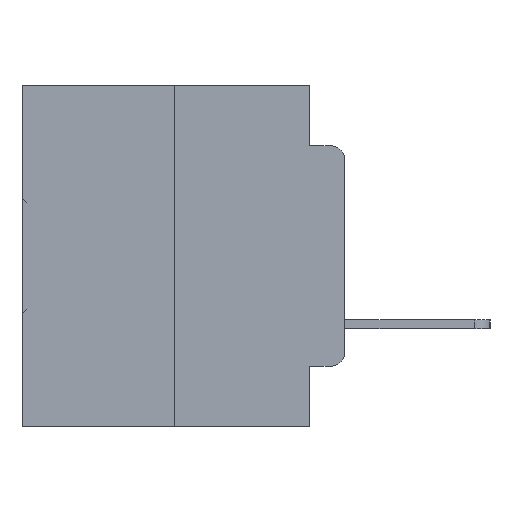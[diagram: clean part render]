
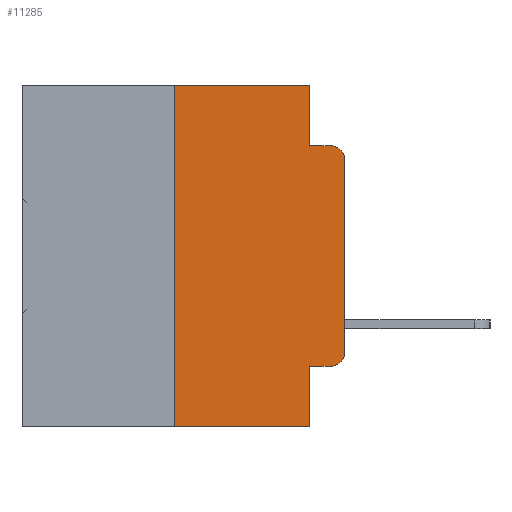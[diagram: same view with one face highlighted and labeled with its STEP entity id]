
A CAD part, left-side view. The second image highlights one B-rep face of the part: STEP entity #11285.
In plain terms, the highlighted planar face has unit normal (-1, 0, 0).
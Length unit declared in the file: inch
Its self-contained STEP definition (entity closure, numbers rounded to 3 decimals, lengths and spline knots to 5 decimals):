
#361 = ORIENTED_EDGE ( 'NONE', *, *, #1601, .F. ) ;
#563 = LINE ( 'NONE', #9354, #14780 ) ;
#819 = EDGE_CURVE ( 'NONE', #1945, #3433, #21607, .T. ) ;
#1034 = EDGE_CURVE ( 'NONE', #19495, #1432, #10415, .T. ) ;
#1432 = VERTEX_POINT ( 'NONE', #14730 ) ;
#1601 = EDGE_CURVE ( 'NONE', #3023, #9306, #14296, .T. ) ;
#1721 = ORIENTED_EDGE ( 'NONE', *, *, #4507, .F. ) ;
#1945 = VERTEX_POINT ( 'NONE', #17935 ) ;
#2360 = DIRECTION ( 'NONE',  ( 0., 0., -1. ) ) ;
#3023 = VERTEX_POINT ( 'NONE', #15230 ) ;
#3433 = VERTEX_POINT ( 'NONE', #30194 ) ;
#3732 = PLANE ( 'NONE',  #27382 ) ;
#4284 = DIRECTION ( 'NONE',  ( 0., -1., 0. ) ) ;
#4507 = EDGE_CURVE ( 'NONE', #1432, #3023, #7591, .T. ) ;
#4677 = EDGE_CURVE ( 'NONE', #1945, #15391, #12441, .T. ) ;
#4767 = VECTOR ( 'NONE', #4284, 39.37008 ) ;
#5169 = CIRCLE ( 'NONE', #24765, 0.02 ) ;
#5280 = CARTESIAN_POINT ( 'NONE',  ( 0., 0.473, 0. ) ) ;
#6507 = DIRECTION ( 'NONE',  ( 1., 0., 0. ) ) ;
#6727 = VERTEX_POINT ( 'NONE', #6832 ) ;
#6832 = CARTESIAN_POINT ( 'NONE',  ( 0., 0., -0.1085 ) ) ;
#7591 = LINE ( 'NONE', #5280, #20413 ) ;
#7931 = DIRECTION ( 'NONE',  ( 0., -1., 0. ) ) ;
#9306 = VERTEX_POINT ( 'NONE', #15198 ) ;
#9354 = CARTESIAN_POINT ( 'NONE',  ( 0., 0., 0. ) ) ;
#9604 = CARTESIAN_POINT ( 'NONE',  ( 0., 0.02, -0.3915 ) ) ;
#9693 = LINE ( 'NONE', #28552, #29025 ) ;
#9875 = VERTEX_POINT ( 'NONE', #10450 ) ;
#10415 = LINE ( 'NONE', #16819, #16546 ) ;
#10450 = CARTESIAN_POINT ( 'NONE',  ( 0., 0., -0.3915 ) ) ;
#10580 = DIRECTION ( 'NONE',  ( 0., 0., -1. ) ) ;
#10961 = DIRECTION ( 'NONE',  ( 0., -1., 0. ) ) ;
#11285 = ADVANCED_FACE ( 'NONE', ( #14634 ), #3732, .F. ) ;
#11453 = EDGE_CURVE ( 'NONE', #9306, #14674, #9693, .T. ) ;
#12220 = DIRECTION ( 'NONE',  ( 0., 0., -1. ) ) ;
#12441 = LINE ( 'NONE', #16809, #25071 ) ;
#13444 = VECTOR ( 'NONE', #10580, 39.37008 ) ;
#13806 = CARTESIAN_POINT ( 'NONE',  ( 0., 0.473, 0. ) ) ;
#14182 = EDGE_CURVE ( 'NONE', #9875, #6727, #563, .T. ) ;
#14296 = LINE ( 'NONE', #33004, #13444 ) ;
#14634 = FACE_OUTER_BOUND ( 'NONE', #26899, .T. ) ;
#14674 = VERTEX_POINT ( 'NONE', #29886 ) ;
#14727 = DIRECTION ( 'NONE',  ( 0., -1., 0. ) ) ;
#14730 = CARTESIAN_POINT ( 'NONE',  ( 0., 0.25, 0. ) ) ;
#14780 = VECTOR ( 'NONE', #24565, 39.37008 ) ;
#15198 = CARTESIAN_POINT ( 'NONE',  ( 0., 0.051, -0.0885 ) ) ;
#15230 = CARTESIAN_POINT ( 'NONE',  ( 0., 0.051, 0. ) ) ;
#15391 = VERTEX_POINT ( 'NONE', #27824 ) ;
#16546 = VECTOR ( 'NONE', #18777, 39.37008 ) ;
#16809 = CARTESIAN_POINT ( 'NONE',  ( 0., 0.051, 0. ) ) ;
#16819 = CARTESIAN_POINT ( 'NONE',  ( 0., 0.25, 0. ) ) ;
#17055 = EDGE_CURVE ( 'NONE', #19495, #15391, #30967, .T. ) ;
#17480 = AXIS2_PLACEMENT_3D ( 'NONE', #32906, #18168, #2360 ) ;
#17935 = CARTESIAN_POINT ( 'NONE',  ( 0., 0.051, -0.4115 ) ) ;
#18168 = DIRECTION ( 'NONE',  ( -1., 0., 0. ) ) ;
#18777 = DIRECTION ( 'NONE',  ( 0., 0., 1. ) ) ;
#19151 = ORIENTED_EDGE ( 'NONE', *, *, #11453, .F. ) ;
#19283 = DIRECTION ( 'NONE',  ( 0., 0., -1. ) ) ;
#19495 = VERTEX_POINT ( 'NONE', #29749 ) ;
#19832 = CARTESIAN_POINT ( 'NONE',  ( 0., 0.473, -0.5 ) ) ;
#20413 = VECTOR ( 'NONE', #7931, 39.37008 ) ;
#20563 = ORIENTED_EDGE ( 'NONE', *, *, #819, .T. ) ;
#20808 = VECTOR ( 'NONE', #14727, 39.37008 ) ;
#21006 = EDGE_CURVE ( 'NONE', #6727, #14674, #28845, .T. ) ;
#21161 = ORIENTED_EDGE ( 'NONE', *, *, #21006, .T. ) ;
#21607 = LINE ( 'NONE', #23206, #20808 ) ;
#23206 = CARTESIAN_POINT ( 'NONE',  ( 0., 0.051, -0.4115 ) ) ;
#24333 = DIRECTION ( 'NONE',  ( 0., 0., -1. ) ) ;
#24565 = DIRECTION ( 'NONE',  ( 0., 0., 1. ) ) ;
#24678 = EDGE_CURVE ( 'NONE', #3433, #9875, #5169, .T. ) ;
#24765 = AXIS2_PLACEMENT_3D ( 'NONE', #9604, #27270, #12220 ) ;
#25071 = VECTOR ( 'NONE', #19283, 39.37008 ) ;
#25306 = ORIENTED_EDGE ( 'NONE', *, *, #24678, .T. ) ;
#25459 = ORIENTED_EDGE ( 'NONE', *, *, #17055, .T. ) ;
#25636 = ORIENTED_EDGE ( 'NONE', *, *, #1034, .F. ) ;
#26899 = EDGE_LOOP ( 'NONE', ( #28018, #21161, #19151, #361, #1721, #25636, #25459, #27468, #20563, #25306 ) ) ;
#27270 = DIRECTION ( 'NONE',  ( -1., 0., 0. ) ) ;
#27382 = AXIS2_PLACEMENT_3D ( 'NONE', #13806, #6507, #24333 ) ;
#27468 = ORIENTED_EDGE ( 'NONE', *, *, #4677, .F. ) ;
#27824 = CARTESIAN_POINT ( 'NONE',  ( 0., 0.051, -0.5 ) ) ;
#28018 = ORIENTED_EDGE ( 'NONE', *, *, #14182, .T. ) ;
#28552 = CARTESIAN_POINT ( 'NONE',  ( 0., 0.051, -0.0885 ) ) ;
#28845 = CIRCLE ( 'NONE', #17480, 0.02 ) ;
#29025 = VECTOR ( 'NONE', #10961, 39.37008 ) ;
#29749 = CARTESIAN_POINT ( 'NONE',  ( 0., 0.25, -0.5 ) ) ;
#29886 = CARTESIAN_POINT ( 'NONE',  ( 0., 0.02, -0.0885 ) ) ;
#30194 = CARTESIAN_POINT ( 'NONE',  ( 0., 0.02, -0.4115 ) ) ;
#30967 = LINE ( 'NONE', #19832, #4767 ) ;
#32906 = CARTESIAN_POINT ( 'NONE',  ( 0., 0.02, -0.1085 ) ) ;
#33004 = CARTESIAN_POINT ( 'NONE',  ( 0., 0.051, 0. ) ) ;
